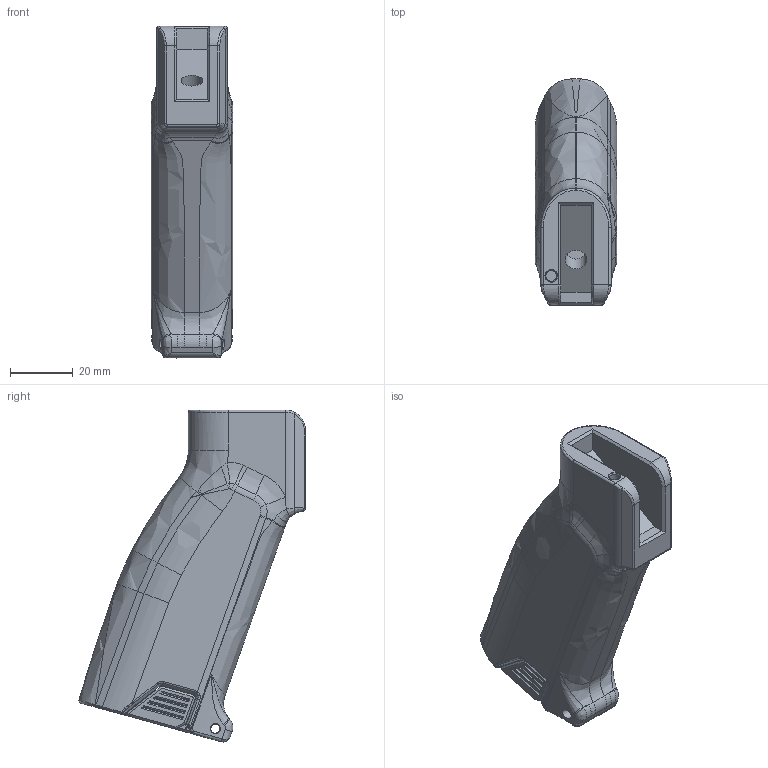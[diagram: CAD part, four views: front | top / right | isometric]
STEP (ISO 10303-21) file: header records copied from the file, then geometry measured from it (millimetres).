
FILE_DESCRIPTION(/* description */ (''),/* implementation_level */ '2;1');
FILE_NAME(/* name */ 'Full Grip Concept.step',/* time_stamp */ '2021-05-07T03:05:05-04:00',/* author */ (''),/* organization */ (''),/* preprocessor_version */ 'ST-DEVELOPER v18.1',/* originating_system */ 'Autodesk Translation Framework v10.6.0.1341',/* authorisation */ '');
FILE_SCHEMA (('AUTOMOTIVE_DESIGN { 1 0 10303 214 3 1 1 }'));
Length unit declared in the file: millimetre
Products named in the file (1): Full Grip Concept
Bounding box: 25.93 x 72.09 x 105.63 mm (x, y, z)
Volume: 44892.7 mm3; surface area: 25667.3 mm2
Topology: 2 solids, 2 shells, 824 faces, 2063 edges, 1207 vertices
Faces by surface type: bspline 372, plane 218, cylinder 183, cone 32, torus 17, sphere 2
Full cylindrical faces by diameter (mm): 2.9 x1, 3.2 x2, 3.4 x1, 6.8 x1, 11.221 x1, 12.721 x1
Entity records: 33884 total; most frequent: CARTESIAN_POINT 16744, ORIENTED_EDGE 4026, DIRECTION 2748, EDGE_CURVE 2013, VERTEX_POINT 1207, AXIS2_PLACEMENT_3D 981, EDGE_LOOP 846, FACE_OUTER_BOUND 824
